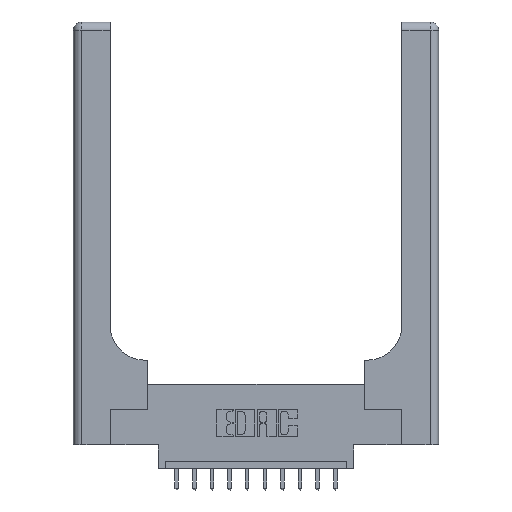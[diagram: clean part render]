
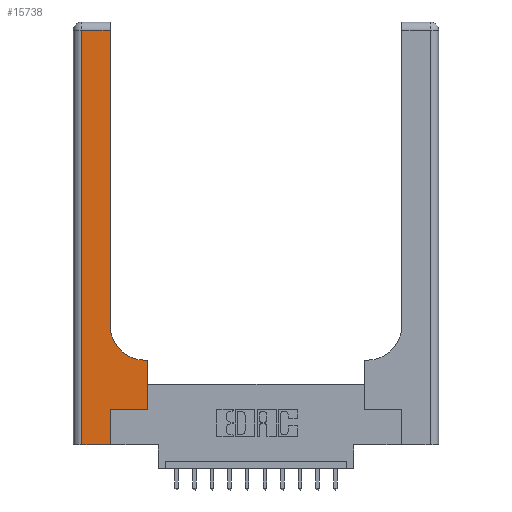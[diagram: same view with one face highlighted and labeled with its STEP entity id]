
A CAD part, top view. The second image highlights one B-rep face of the part: STEP entity #15738.
In plain terms, the highlighted planar face has unit normal (0, 0, 1).
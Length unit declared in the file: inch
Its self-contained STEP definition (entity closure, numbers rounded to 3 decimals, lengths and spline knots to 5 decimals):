
#19 = CIRCLE ( 'NONE', #15515, 0.25 ) ;
#34 = LINE ( 'NONE', #5246, #7939 ) ;
#69 = ORIENTED_EDGE ( 'NONE', *, *, #13084, .T. ) ;
#343 = EDGE_CURVE ( 'NONE', #6235, #12110, #16185, .T. ) ;
#928 = LINE ( 'NONE', #3171, #2160 ) ;
#974 = VECTOR ( 'NONE', #5258, 39.37008 ) ;
#1436 = CARTESIAN_POINT ( 'NONE',  ( 0.26, 2.94, 0.37 ) ) ;
#1787 = DIRECTION ( 'NONE',  ( 1., 0., 0. ) ) ;
#2160 = VECTOR ( 'NONE', #9592, 39.37008 ) ;
#3171 = CARTESIAN_POINT ( 'NONE',  ( 0.06, 3., 0.37 ) ) ;
#3399 = CARTESIAN_POINT ( 'NONE',  ( 0.528, 0.25, 0.37 ) ) ;
#3645 = LINE ( 'NONE', #13889, #9087 ) ;
#3731 = VECTOR ( 'NONE', #5789, 39.37008 ) ;
#3733 = DIRECTION ( 'NONE',  ( -1., 0., 0. ) ) ;
#3745 = EDGE_CURVE ( 'NONE', #5265, #3815, #10354, .T. ) ;
#3815 = VERTEX_POINT ( 'NONE', #8411 ) ;
#3987 = PLANE ( 'NONE',  #11230 ) ;
#4260 = VERTEX_POINT ( 'NONE', #9458 ) ;
#4526 = VERTEX_POINT ( 'NONE', #12074 ) ;
#4586 = EDGE_CURVE ( 'NONE', #16280, #4260, #928, .T. ) ;
#4669 = ORIENTED_EDGE ( 'NONE', *, *, #14982, .T. ) ;
#5246 = CARTESIAN_POINT ( 'NONE',  ( 0.265, 0.25, 0.37 ) ) ;
#5258 = DIRECTION ( 'NONE',  ( -1., 0., 0. ) ) ;
#5265 = VERTEX_POINT ( 'NONE', #12865 ) ;
#5416 = CARTESIAN_POINT ( 'NONE',  ( 0.51, 0.85, 0.37 ) ) ;
#5581 = EDGE_CURVE ( 'NONE', #3815, #6235, #19, .T. ) ;
#5657 = EDGE_LOOP ( 'NONE', ( #13302, #4669, #13107, #16102, #11312, #69, #15832, #11847, #15721 ) ) ;
#5789 = DIRECTION ( 'NONE',  ( 0., 1., 0. ) ) ;
#6015 = VERTEX_POINT ( 'NONE', #3399 ) ;
#6038 = EDGE_CURVE ( 'NONE', #6015, #5265, #6967, .T. ) ;
#6235 = VERTEX_POINT ( 'NONE', #12712 ) ;
#6304 = VECTOR ( 'NONE', #8804, 39.37008 ) ;
#6484 = DIRECTION ( 'NONE',  ( -1., 0., 0. ) ) ;
#6967 = LINE ( 'NONE', #9422, #3731 ) ;
#7096 = CARTESIAN_POINT ( 'NONE',  ( 0.06, 2.94, 0.37 ) ) ;
#7485 = CARTESIAN_POINT ( 'NONE',  ( 0.265, 0., 0.37 ) ) ;
#7939 = VECTOR ( 'NONE', #15171, 39.37008 ) ;
#8411 = CARTESIAN_POINT ( 'NONE',  ( 0.51, 0.6, 0.37 ) ) ;
#8646 = CARTESIAN_POINT ( 'NONE',  ( 0.26, 3., 0.37 ) ) ;
#8804 = DIRECTION ( 'NONE',  ( 0., 1., 0. ) ) ;
#9087 = VECTOR ( 'NONE', #3733, 39.37008 ) ;
#9422 = CARTESIAN_POINT ( 'NONE',  ( 0.528, 0.25, 0.37 ) ) ;
#9458 = CARTESIAN_POINT ( 'NONE',  ( 0.06, 0., 0.37 ) ) ;
#9592 = DIRECTION ( 'NONE',  ( 0., -1., 0. ) ) ;
#10295 = LINE ( 'NONE', #12784, #12361 ) ;
#10354 = LINE ( 'NONE', #14097, #974 ) ;
#11230 = AXIS2_PLACEMENT_3D ( 'NONE', #16239, #13983, #6484 ) ;
#11237 = EDGE_CURVE ( 'NONE', #4260, #14778, #10295, .T. ) ;
#11312 = ORIENTED_EDGE ( 'NONE', *, *, #12684, .T. ) ;
#11847 = ORIENTED_EDGE ( 'NONE', *, *, #3745, .T. ) ;
#12058 = CARTESIAN_POINT ( 'NONE',  ( 0.265, 0., 0.37 ) ) ;
#12074 = CARTESIAN_POINT ( 'NONE',  ( 0.265, 0.25, 0.37 ) ) ;
#12110 = VERTEX_POINT ( 'NONE', #1436 ) ;
#12150 = VECTOR ( 'NONE', #13211, 39.37008 ) ;
#12361 = VECTOR ( 'NONE', #1787, 39.37008 ) ;
#12684 = EDGE_CURVE ( 'NONE', #14778, #4526, #13448, .T. ) ;
#12712 = CARTESIAN_POINT ( 'NONE',  ( 0.26, 0.85, 0.37 ) ) ;
#12784 = CARTESIAN_POINT ( 'NONE',  ( 0., 0., 0.37 ) ) ;
#12828 = DIRECTION ( 'NONE',  ( 0., 0., -1. ) ) ;
#12865 = CARTESIAN_POINT ( 'NONE',  ( 0.528, 0.6, 0.37 ) ) ;
#13084 = EDGE_CURVE ( 'NONE', #4526, #6015, #34, .T. ) ;
#13107 = ORIENTED_EDGE ( 'NONE', *, *, #4586, .T. ) ;
#13211 = DIRECTION ( 'NONE',  ( 0., 1., 0. ) ) ;
#13302 = ORIENTED_EDGE ( 'NONE', *, *, #343, .T. ) ;
#13448 = LINE ( 'NONE', #12058, #12150 ) ;
#13889 = CARTESIAN_POINT ( 'NONE',  ( 0., 2.94, 0.37 ) ) ;
#13902 = FACE_OUTER_BOUND ( 'NONE', #5657, .T. ) ;
#13983 = DIRECTION ( 'NONE',  ( 0., 0., -1. ) ) ;
#14097 = CARTESIAN_POINT ( 'NONE',  ( 0.26, 0.6, 0.37 ) ) ;
#14778 = VERTEX_POINT ( 'NONE', #7485 ) ;
#14982 = EDGE_CURVE ( 'NONE', #12110, #16280, #3645, .T. ) ;
#15171 = DIRECTION ( 'NONE',  ( 1., 0., 0. ) ) ;
#15408 = DIRECTION ( 'NONE',  ( 1., 0., 0. ) ) ;
#15515 = AXIS2_PLACEMENT_3D ( 'NONE', #5416, #12828, #15408 ) ;
#15721 = ORIENTED_EDGE ( 'NONE', *, *, #5581, .T. ) ;
#15738 = ADVANCED_FACE ( 'NONE', ( #13902 ), #3987, .F. ) ;
#15832 = ORIENTED_EDGE ( 'NONE', *, *, #6038, .T. ) ;
#16102 = ORIENTED_EDGE ( 'NONE', *, *, #11237, .T. ) ;
#16185 = LINE ( 'NONE', #8646, #6304 ) ;
#16239 = CARTESIAN_POINT ( 'NONE',  ( 0., 3., 0.37 ) ) ;
#16280 = VERTEX_POINT ( 'NONE', #7096 ) ;
